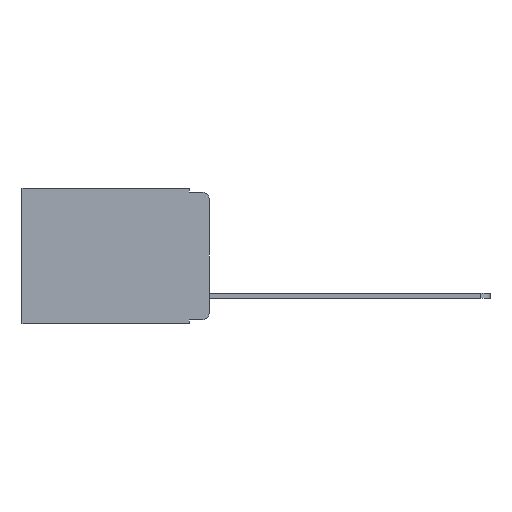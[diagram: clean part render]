
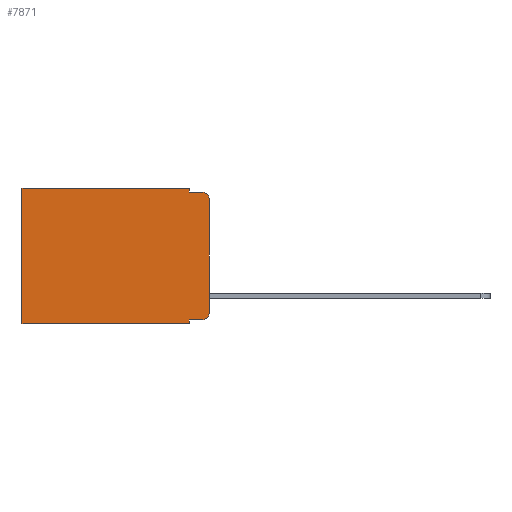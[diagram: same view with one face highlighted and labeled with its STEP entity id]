
A CAD part, left-side view. The second image highlights one B-rep face of the part: STEP entity #7871.
In plain terms, the highlighted planar face has unit normal (-1, 0, 0).
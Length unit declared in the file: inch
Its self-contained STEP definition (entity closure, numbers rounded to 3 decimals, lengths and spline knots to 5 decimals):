
#77 = DIRECTION ( 'NONE',  ( 0., 0., -1. ) ) ;
#173 = DIRECTION ( 'NONE',  ( 0., 1., 0. ) ) ;
#252 = LINE ( 'NONE', #7400, #7529 ) ;
#263 = VECTOR ( 'NONE', #77, 39.37008 ) ;
#382 = VERTEX_POINT ( 'NONE', #4280 ) ;
#385 = VERTEX_POINT ( 'NONE', #5777 ) ;
#480 = LINE ( 'NONE', #1990, #9033 ) ;
#542 = CARTESIAN_POINT ( 'NONE',  ( 0.298, 0.473, 0. ) ) ;
#544 = LINE ( 'NONE', #6081, #263 ) ;
#581 = CARTESIAN_POINT ( 'NONE',  ( 0.298, 0., 0. ) ) ;
#737 = ORIENTED_EDGE ( 'NONE', *, *, #5066, .F. ) ;
#818 = EDGE_CURVE ( 'NONE', #5128, #6239, #8292, .T. ) ;
#1229 = AXIS2_PLACEMENT_3D ( 'NONE', #2646, #8321, #3526 ) ;
#1307 = ORIENTED_EDGE ( 'NONE', *, *, #5496, .T. ) ;
#1514 = CARTESIAN_POINT ( 'NONE',  ( 0.298, 0.051, -0.01 ) ) ;
#1527 = CIRCLE ( 'NONE', #1229, 0.02 ) ;
#1626 = VECTOR ( 'NONE', #10359, 39.37008 ) ;
#1990 = CARTESIAN_POINT ( 'NONE',  ( 0.298, 0.051, -0.01 ) ) ;
#2031 = CARTESIAN_POINT ( 'NONE',  ( 0.298, 0.02, -0.333 ) ) ;
#2330 = CIRCLE ( 'NONE', #10585, 0.02 ) ;
#2622 = PLANE ( 'NONE',  #10156 ) ;
#2646 = CARTESIAN_POINT ( 'NONE',  ( 0.298, 0.02, -0.03 ) ) ;
#3126 = ORIENTED_EDGE ( 'NONE', *, *, #818, .T. ) ;
#3247 = DIRECTION ( 'NONE',  ( 0., 0., -1. ) ) ;
#3359 = CARTESIAN_POINT ( 'NONE',  ( 0.298, 0.02, -0.01 ) ) ;
#3494 = DIRECTION ( 'NONE',  ( 0., 0., -1. ) ) ;
#3526 = DIRECTION ( 'NONE',  ( 0., 0., -1. ) ) ;
#3631 = CARTESIAN_POINT ( 'NONE',  ( 0.298, 0.473, 0. ) ) ;
#3691 = CARTESIAN_POINT ( 'NONE',  ( 0.298, 0.051, -0.333 ) ) ;
#3858 = CARTESIAN_POINT ( 'NONE',  ( 0.298, 0.051, 0. ) ) ;
#4280 = CARTESIAN_POINT ( 'NONE',  ( 0.298, 0., -0.313 ) ) ;
#5023 = CARTESIAN_POINT ( 'NONE',  ( 0.298, 0.02, -0.313 ) ) ;
#5066 = EDGE_CURVE ( 'NONE', #5128, #7688, #544, .T. ) ;
#5128 = VERTEX_POINT ( 'NONE', #3691 ) ;
#5161 = CARTESIAN_POINT ( 'NONE',  ( 0.298, 0.051, -0.333 ) ) ;
#5496 = EDGE_CURVE ( 'NONE', #7721, #7310, #252, .T. ) ;
#5580 = ORIENTED_EDGE ( 'NONE', *, *, #9121, .T. ) ;
#5613 = EDGE_CURVE ( 'NONE', #9114, #6546, #1527, .T. ) ;
#5759 = EDGE_CURVE ( 'NONE', #7688, #385, #8711, .T. ) ;
#5777 = CARTESIAN_POINT ( 'NONE',  ( 0.298, 0.473, -0.343 ) ) ;
#5843 = ORIENTED_EDGE ( 'NONE', *, *, #10562, .F. ) ;
#5851 = DIRECTION ( 'NONE',  ( 0., 0., -1. ) ) ;
#6079 = VECTOR ( 'NONE', #8655, 39.37008 ) ;
#6081 = CARTESIAN_POINT ( 'NONE',  ( 0.298, 0.051, 0. ) ) ;
#6237 = VECTOR ( 'NONE', #8061, 39.37008 ) ;
#6239 = VERTEX_POINT ( 'NONE', #2031 ) ;
#6473 = ORIENTED_EDGE ( 'NONE', *, *, #7049, .F. ) ;
#6524 = CARTESIAN_POINT ( 'NONE',  ( 0.298, 0., -0.03 ) ) ;
#6546 = VERTEX_POINT ( 'NONE', #3359 ) ;
#6660 = VECTOR ( 'NONE', #173, 39.37008 ) ;
#6860 = LINE ( 'NONE', #542, #10216 ) ;
#7049 = EDGE_CURVE ( 'NONE', #9114, #382, #8210, .T. ) ;
#7310 = VERTEX_POINT ( 'NONE', #3631 ) ;
#7337 = ORIENTED_EDGE ( 'NONE', *, *, #5613, .T. ) ;
#7371 = CARTESIAN_POINT ( 'NONE',  ( 0.298, 0.051, 0. ) ) ;
#7400 = CARTESIAN_POINT ( 'NONE',  ( 0.298, 0., 0. ) ) ;
#7529 = VECTOR ( 'NONE', #8167, 39.37008 ) ;
#7688 = VERTEX_POINT ( 'NONE', #10381 ) ;
#7707 = ORIENTED_EDGE ( 'NONE', *, *, #5759, .F. ) ;
#7721 = VERTEX_POINT ( 'NONE', #7371 ) ;
#7871 = ADVANCED_FACE ( 'NONE', ( #9154 ), #2622, .F. ) ;
#8061 = DIRECTION ( 'NONE',  ( 0., -1., 0. ) ) ;
#8100 = EDGE_CURVE ( 'NONE', #8382, #6546, #480, .T. ) ;
#8167 = DIRECTION ( 'NONE',  ( 0., 1., 0. ) ) ;
#8170 = LINE ( 'NONE', #3858, #6079 ) ;
#8210 = LINE ( 'NONE', #581, #1626 ) ;
#8292 = LINE ( 'NONE', #5161, #6237 ) ;
#8293 = DIRECTION ( 'NONE',  ( 1., 0., 0. ) ) ;
#8321 = DIRECTION ( 'NONE',  ( -1., 0., 0. ) ) ;
#8382 = VERTEX_POINT ( 'NONE', #1514 ) ;
#8478 = CARTESIAN_POINT ( 'NONE',  ( 0.298, 0., -0.343 ) ) ;
#8655 = DIRECTION ( 'NONE',  ( 0., 0., -1. ) ) ;
#8711 = LINE ( 'NONE', #8478, #6660 ) ;
#8777 = ORIENTED_EDGE ( 'NONE', *, *, #8100, .F. ) ;
#9033 = VECTOR ( 'NONE', #9268, 39.37008 ) ;
#9114 = VERTEX_POINT ( 'NONE', #6524 ) ;
#9121 = EDGE_CURVE ( 'NONE', #7310, #385, #6860, .T. ) ;
#9154 = FACE_OUTER_BOUND ( 'NONE', #9430, .T. ) ;
#9268 = DIRECTION ( 'NONE',  ( 0., -1., 0. ) ) ;
#9318 = EDGE_CURVE ( 'NONE', #6239, #382, #2330, .T. ) ;
#9430 = EDGE_LOOP ( 'NONE', ( #6473, #7337, #8777, #5843, #1307, #5580, #7707, #737, #3126, #10549 ) ) ;
#9806 = CARTESIAN_POINT ( 'NONE',  ( 0.298, 0., 0. ) ) ;
#10156 = AXIS2_PLACEMENT_3D ( 'NONE', #9806, #8293, #3494 ) ;
#10216 = VECTOR ( 'NONE', #3247, 39.37008 ) ;
#10359 = DIRECTION ( 'NONE',  ( 0., 0., -1. ) ) ;
#10381 = CARTESIAN_POINT ( 'NONE',  ( 0.298, 0.051, -0.343 ) ) ;
#10457 = DIRECTION ( 'NONE',  ( -1., 0., 0. ) ) ;
#10549 = ORIENTED_EDGE ( 'NONE', *, *, #9318, .T. ) ;
#10562 = EDGE_CURVE ( 'NONE', #7721, #8382, #8170, .T. ) ;
#10585 = AXIS2_PLACEMENT_3D ( 'NONE', #5023, #10457, #5851 ) ;
